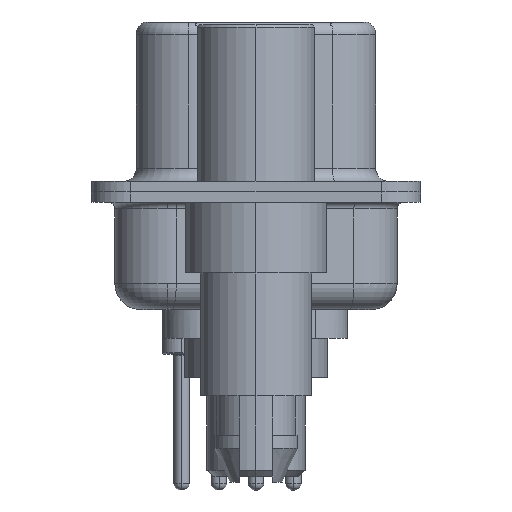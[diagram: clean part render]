
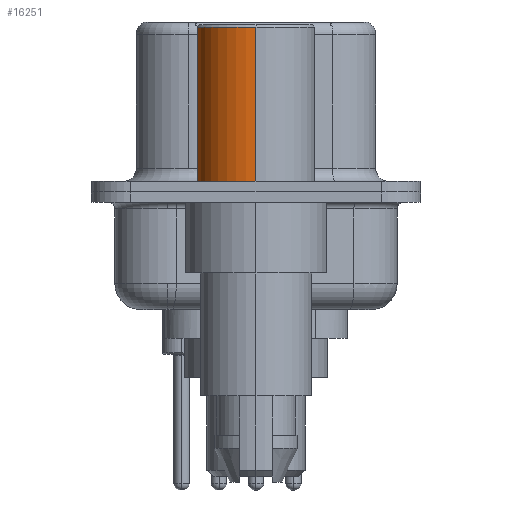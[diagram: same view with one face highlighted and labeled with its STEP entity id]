
A CAD part, left-side view. The second image highlights one B-rep face of the part: STEP entity #16251.
In plain terms, the highlighted cylindrical face has radius 2.25 mm (diameter 4.5 mm), a partial arc.
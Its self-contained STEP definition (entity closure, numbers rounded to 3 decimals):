
#58 = CARTESIAN_POINT ( 'NONE',  ( 2.25, 0., 6.3 ) ) ;
#168 = ORIENTED_EDGE ( 'NONE', *, *, #19309, .F. ) ;
#343 = AXIS2_PLACEMENT_3D ( 'NONE', #478, #11487, #2070 ) ;
#478 = CARTESIAN_POINT ( 'NONE',  ( 0., 0., 6.3 ) ) ;
#604 = FACE_OUTER_BOUND ( 'NONE', #16365, .T. ) ;
#783 = CARTESIAN_POINT ( 'NONE',  ( 0., 0., 0.4 ) ) ;
#973 = CIRCLE ( 'NONE', #15441, 2.25 ) ;
#1638 = VECTOR ( 'NONE', #18159, 1000. ) ;
#2070 = DIRECTION ( 'NONE',  ( 1., 0., 0. ) ) ;
#2370 = DIRECTION ( 'NONE',  ( 1., 0., 0. ) ) ;
#3176 = EDGE_CURVE ( 'NONE', #7134, #6095, #13859, .T. ) ;
#3997 = DIRECTION ( 'NONE',  ( 0., 0., 1. ) ) ;
#4302 = VERTEX_POINT ( 'NONE', #17156 ) ;
#5923 = CARTESIAN_POINT ( 'NONE',  ( -2.25, 0., 6.3 ) ) ;
#6095 = VERTEX_POINT ( 'NONE', #5923 ) ;
#6337 = DIRECTION ( 'NONE',  ( 1., 0., 0. ) ) ;
#7134 = VERTEX_POINT ( 'NONE', #14832 ) ;
#7366 = ORIENTED_EDGE ( 'NONE', *, *, #14273, .F. ) ;
#7600 = CIRCLE ( 'NONE', #343, 2.25 ) ;
#8162 = AXIS2_PLACEMENT_3D ( 'NONE', #16015, #12710, #6337 ) ;
#8380 = EDGE_CURVE ( 'NONE', #4302, #7134, #973, .T. ) ;
#8725 = VECTOR ( 'NONE', #3997, 1000. ) ;
#10208 = CARTESIAN_POINT ( 'NONE',  ( 2.25, 0., 0.581 ) ) ;
#10410 = ORIENTED_EDGE ( 'NONE', *, *, #3176, .T. ) ;
#11487 = DIRECTION ( 'NONE',  ( 0., 0., 1. ) ) ;
#11791 = DIRECTION ( 'NONE',  ( 0., 0., 1. ) ) ;
#12710 = DIRECTION ( 'NONE',  ( 0., 0., 1. ) ) ;
#12729 = CYLINDRICAL_SURFACE ( 'NONE', #8162, 2.25 ) ;
#12796 = ORIENTED_EDGE ( 'NONE', *, *, #8380, .T. ) ;
#13044 = LINE ( 'NONE', #10208, #8725 ) ;
#13859 = LINE ( 'NONE', #14946, #1638 ) ;
#14273 = EDGE_CURVE ( 'NONE', #4302, #17455, #13044, .T. ) ;
#14832 = CARTESIAN_POINT ( 'NONE',  ( -2.25, 0., 0.4 ) ) ;
#14946 = CARTESIAN_POINT ( 'NONE',  ( -2.25, 0., 0.581 ) ) ;
#15441 = AXIS2_PLACEMENT_3D ( 'NONE', #783, #11791, #2370 ) ;
#16015 = CARTESIAN_POINT ( 'NONE',  ( 0., 0., 0.581 ) ) ;
#16251 = ADVANCED_FACE ( 'NONE', ( #604 ), #12729, .T. ) ;
#16365 = EDGE_LOOP ( 'NONE', ( #12796, #10410, #168, #7366 ) ) ;
#17156 = CARTESIAN_POINT ( 'NONE',  ( 2.25, 0., 0.4 ) ) ;
#17455 = VERTEX_POINT ( 'NONE', #58 ) ;
#18159 = DIRECTION ( 'NONE',  ( 0., 0., 1. ) ) ;
#19309 = EDGE_CURVE ( 'NONE', #17455, #6095, #7600, .T. ) ;
